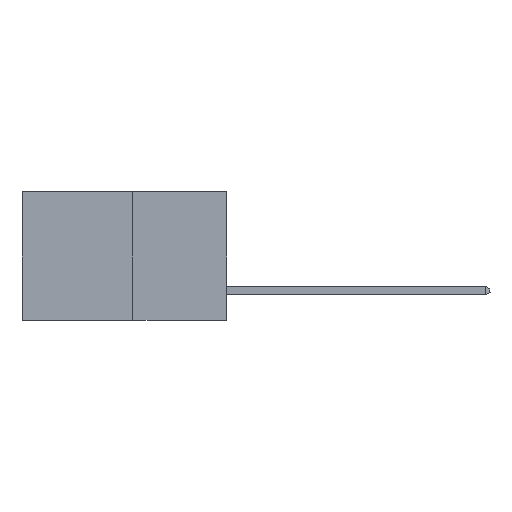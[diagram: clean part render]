
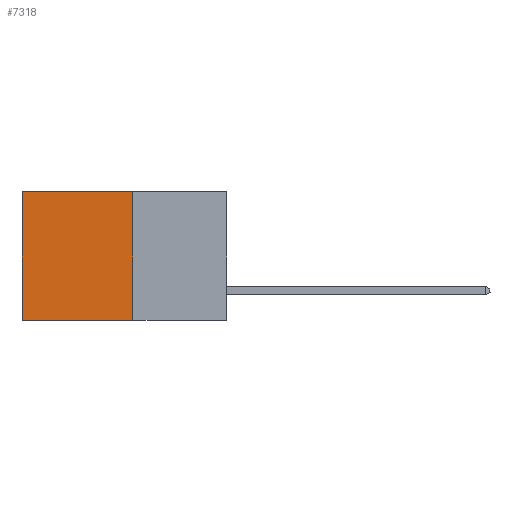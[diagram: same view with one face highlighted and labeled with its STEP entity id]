
A CAD part, left-side view. The second image highlights one B-rep face of the part: STEP entity #7318.
In plain terms, the highlighted planar face has unit normal (-1, 0, 0).
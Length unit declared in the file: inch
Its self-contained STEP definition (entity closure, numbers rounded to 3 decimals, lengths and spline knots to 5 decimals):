
#681 = LINE ( 'NONE', #9757, #17258 ) ;
#721 = VECTOR ( 'NONE', #2601, 39.37008 ) ;
#1043 = AXIS2_PLACEMENT_3D ( 'NONE', #2913, #5654, #15028 ) ;
#2553 = CARTESIAN_POINT ( 'NONE',  ( 0.277, 0.59, 0. ) ) ;
#2601 = DIRECTION ( 'NONE',  ( 0., 1., 0. ) ) ;
#2801 = DIRECTION ( 'NONE',  ( 0., 0., -1. ) ) ;
#2913 = CARTESIAN_POINT ( 'NONE',  ( 0.277, 0.27, -0.37 ) ) ;
#3215 = EDGE_CURVE ( 'NONE', #16536, #10261, #15023, .T. ) ;
#3414 = VERTEX_POINT ( 'NONE', #12612 ) ;
#3733 = CARTESIAN_POINT ( 'NONE',  ( 0.277, 0.59, -0.37 ) ) ;
#4087 = EDGE_CURVE ( 'NONE', #3414, #16536, #8275, .T. ) ;
#4316 = VECTOR ( 'NONE', #2801, 39.37008 ) ;
#4421 = DIRECTION ( 'NONE',  ( 0., 1., 0. ) ) ;
#4520 = FACE_OUTER_BOUND ( 'NONE', #10914, .T. ) ;
#4998 = EDGE_CURVE ( 'NONE', #14005, #10261, #681, .T. ) ;
#5545 = ORIENTED_EDGE ( 'NONE', *, *, #13346, .F. ) ;
#5654 = DIRECTION ( 'NONE',  ( 1., 0., 0. ) ) ;
#7318 = ADVANCED_FACE ( 'NONE', ( #4520 ), #13650, .F. ) ;
#7988 = CARTESIAN_POINT ( 'NONE',  ( 0.277, 0.27, 0. ) ) ;
#8275 = LINE ( 'NONE', #7988, #721 ) ;
#8319 = CARTESIAN_POINT ( 'NONE',  ( 0.277, 0.27, -0.37 ) ) ;
#9757 = CARTESIAN_POINT ( 'NONE',  ( 0.277, 0.27, -0.37 ) ) ;
#10261 = VERTEX_POINT ( 'NONE', #3733 ) ;
#10914 = EDGE_LOOP ( 'NONE', ( #15560, #16923, #5545, #13122 ) ) ;
#11066 = DIRECTION ( 'NONE',  ( 0., 0., -1. ) ) ;
#11287 = CARTESIAN_POINT ( 'NONE',  ( 0.277, 0.27, -0.37 ) ) ;
#12112 = VECTOR ( 'NONE', #11066, 39.37008 ) ;
#12158 = CARTESIAN_POINT ( 'NONE',  ( 0.277, 0.59, -0.37 ) ) ;
#12612 = CARTESIAN_POINT ( 'NONE',  ( 0.277, 0.27, 0. ) ) ;
#13122 = ORIENTED_EDGE ( 'NONE', *, *, #4087, .T. ) ;
#13346 = EDGE_CURVE ( 'NONE', #3414, #14005, #15704, .T. ) ;
#13650 = PLANE ( 'NONE',  #1043 ) ;
#14005 = VERTEX_POINT ( 'NONE', #11287 ) ;
#15023 = LINE ( 'NONE', #12158, #4316 ) ;
#15028 = DIRECTION ( 'NONE',  ( 0., 0., -1. ) ) ;
#15560 = ORIENTED_EDGE ( 'NONE', *, *, #3215, .T. ) ;
#15704 = LINE ( 'NONE', #8319, #12112 ) ;
#16536 = VERTEX_POINT ( 'NONE', #2553 ) ;
#16923 = ORIENTED_EDGE ( 'NONE', *, *, #4998, .F. ) ;
#17258 = VECTOR ( 'NONE', #4421, 39.37008 ) ;
